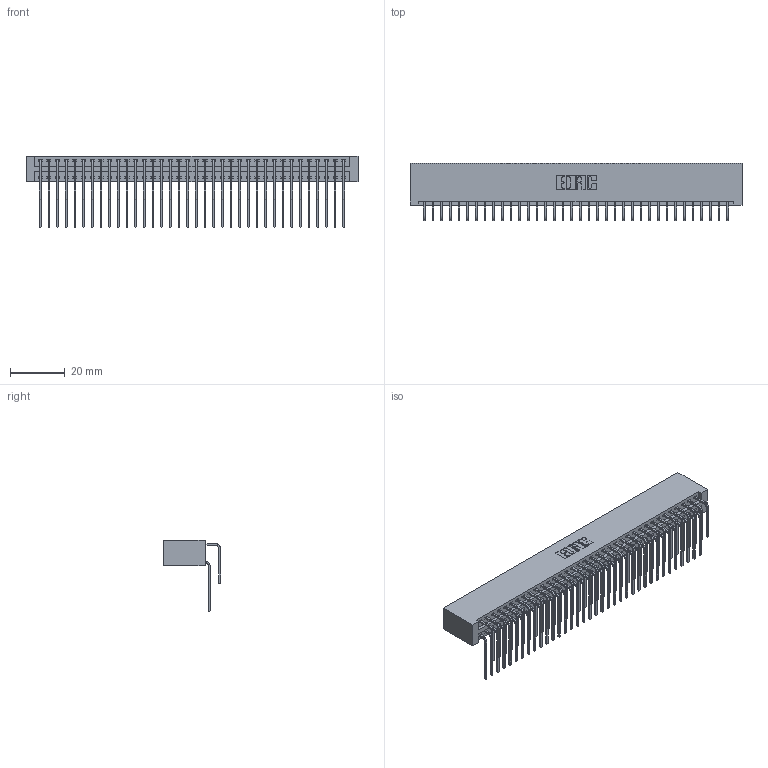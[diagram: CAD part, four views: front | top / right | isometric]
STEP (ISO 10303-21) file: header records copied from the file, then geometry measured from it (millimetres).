
FILE_DESCRIPTION (( 'STEP AP203' ), '1' );
FILE_NAME ('346-072-559-201.STEP', '2022-05-25T00:56:23', ( '' ), ( '' ), 'SwSTEP 2.0', 'SolidWorks 2020', '' );
FILE_SCHEMA (( 'CONFIG_CONTROL_DESIGN' ));
Length unit declared in the file: inch
Products named in the file (4): 345-292-001_559 Tail - 2; 345-292-001_558 559 Tail - 1; 346-072-559-201; 346 Part_No Mounting Lugs
Assembly tree (73 placements, depth 2):
  346-072-559-201
    346 Part_No Mounting Lugs
    345-292-001_558 559 Tail - 1  x36
    345-292-001_559 Tail - 2  x36
Bounding box: 121.54 x 20.89 x 26.16 mm (x, y, z)
Volume: 12793.6 mm3; surface area: 19647.1 mm2
Topology: 73 solids, 73 shells, 4002 faces, 11897 edges, 7834 vertices
Faces by surface type: plane 2736, cylinder 1266
Entity records: 25809 total; most frequent: CARTESIAN_POINT 4311, ORIENTED_EDGE 4194, DIRECTION 3817, EDGE_CURVE 2097, LINE 1789, VECTOR 1789, VERTEX_POINT 1394, AXIS2_PLACEMENT_3D 1014
